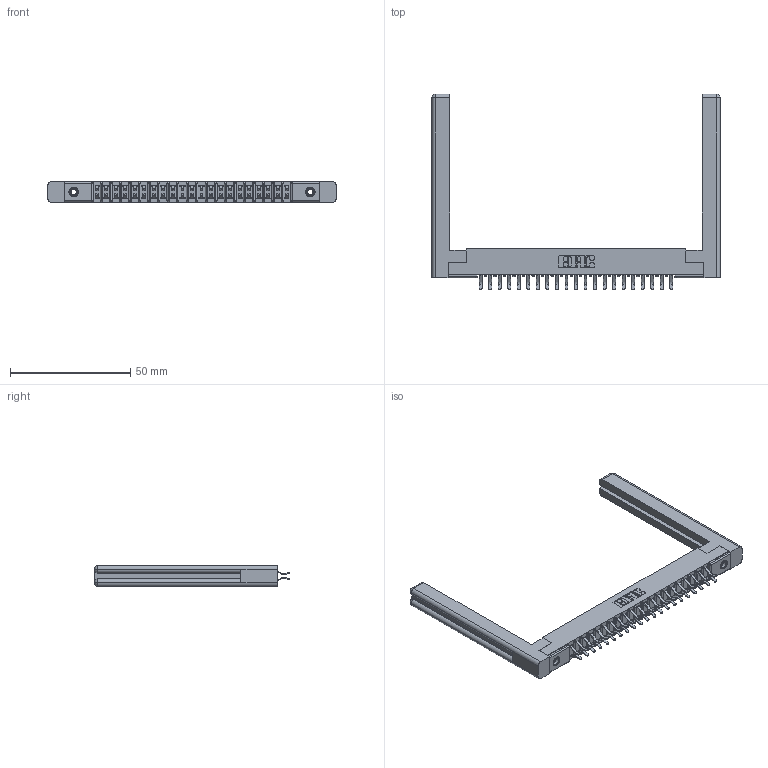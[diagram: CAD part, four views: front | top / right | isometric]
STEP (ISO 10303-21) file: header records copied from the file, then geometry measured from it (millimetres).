
FILE_DESCRIPTION (( 'STEP AP203' ), '1' );
FILE_NAME ('357-042-556-258.STEP', '2019-09-18T06:41:38', ( '' ), ( '' ), 'SwSTEP 2.0', 'SolidWorks 2016', '' );
FILE_SCHEMA (( 'CONFIG_CONTROL_DESIGN' ));
Length unit declared in the file: inch
Products named in the file (5): 307 Part_.156 Dia Mounting Holes; 357-042-556-258; 345-250-001_345-250-001-102; 307-220-058; 307-290-001_556
Assembly tree (47 placements, depth 2):
  357-042-556-258
    307 Part_.156 Dia Mounting Holes
    307-290-001_556  x42
    307-220-058  x2
    345-250-001_345-250-001-102  x2
Bounding box: 119.84 x 81.28 x 8.71 mm (x, y, z)
Volume: 15517.7 mm3; surface area: 18827 mm2
Topology: 47 solids, 47 shells, 2382 faces, 6641 edges, 4298 vertices
Faces by surface type: plane 1540, cylinder 774, sphere 44, torus 12, cone 12
Entity records: 24001 total; most frequent: CARTESIAN_POINT 3952, ORIENTED_EDGE 3856, DIRECTION 3838, EDGE_CURVE 1928, LINE 1466, VECTOR 1466, VERTEX_POINT 1246, AXIS2_PLACEMENT_3D 1186
